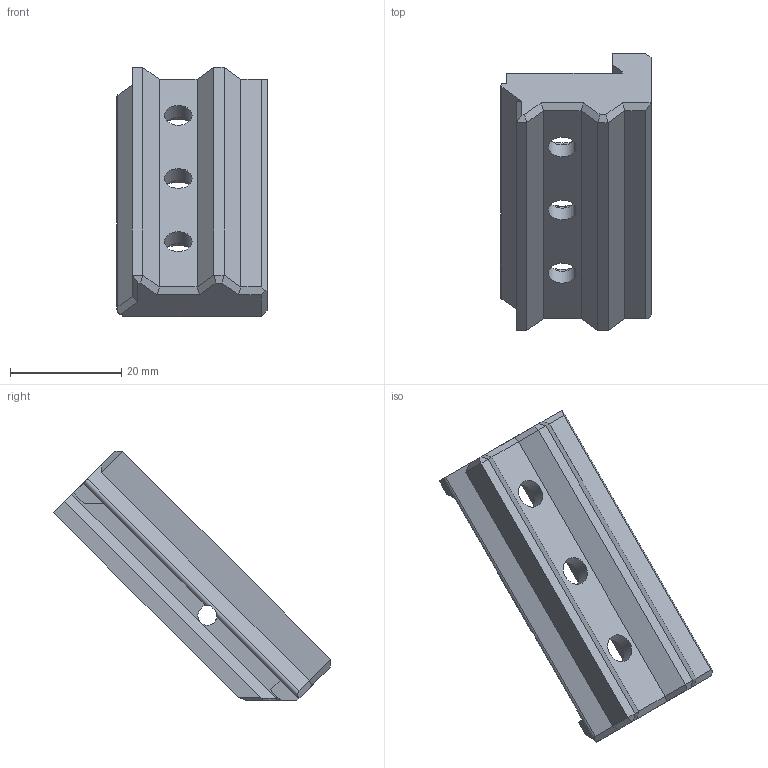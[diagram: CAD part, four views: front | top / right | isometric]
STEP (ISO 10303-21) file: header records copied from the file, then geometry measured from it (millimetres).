
FILE_DESCRIPTION(/* description */ (''),/* implementation_level */ '2;1');
FILE_NAME(/* name */ 'LPL Trijicon Mount 1.175.step',/* time_stamp */ '2023-02-26T20:00:16-06:00',/* author */ (''),/* organization */ (''),/* preprocessor_version */ 'ST-DEVELOPER v19.2',/* originating_system */ 'Autodesk Translation Framework v11.17.0.187',/* authorisation */ '');
FILE_SCHEMA (('AUTOMOTIVE_DESIGN { 1 0 10303 214 3 1 1 }'));
Length unit declared in the file: millimetre
Products named in the file (1): LPL Trijicon Mount (1.175")
Bounding box: 26.93 x 49.68 x 44.69 mm (x, y, z)
Volume: 11237.1 mm3; surface area: 5611.5 mm2
Topology: 1 solids, 1 shells, 72 faces, 187 edges, 118 vertices
Faces by surface type: plane 64, cylinder 8
Full cylindrical faces by diameter (mm): 5 x3, 10 x3
Entity records: 2210 total; most frequent: CARTESIAN_POINT 389, ORIENTED_EDGE 374, DIRECTION 353, EDGE_CURVE 187, LINE 165, VECTOR 165, VERTEX_POINT 118, AXIS2_PLACEMENT_3D 94
